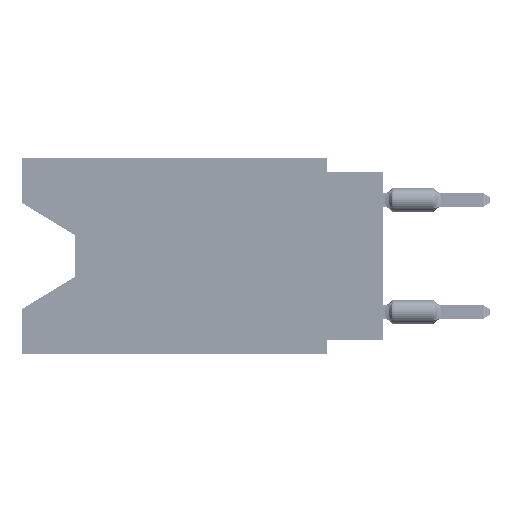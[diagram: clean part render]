
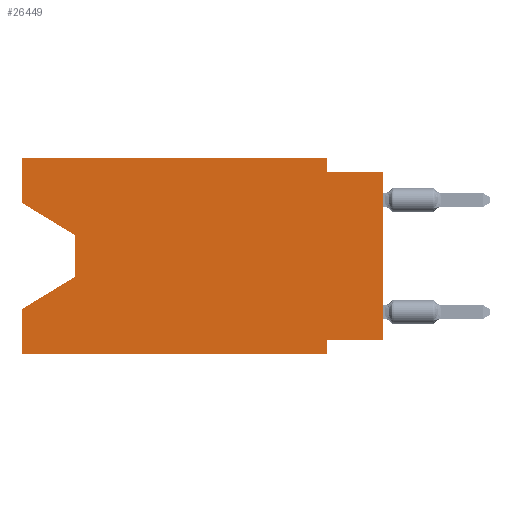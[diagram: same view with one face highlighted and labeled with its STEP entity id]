
A CAD part, left-side view. The second image highlights one B-rep face of the part: STEP entity #26449.
In plain terms, the highlighted planar face has unit normal (-1, 0, 0).
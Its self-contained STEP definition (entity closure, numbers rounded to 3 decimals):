
#415 = EDGE_CURVE ( 'NONE', #91928, #70264, #32800, .T. ) ;
#501 = VECTOR ( 'NONE', #87313, 1000. ) ;
#2110 = VERTEX_POINT ( 'NONE', #8948 ) ;
#2364 = AXIS2_PLACEMENT_3D ( 'NONE', #51618, #16560, #9546 ) ;
#3409 = EDGE_LOOP ( 'NONE', ( #31632, #90401, #66852, #14680, #78663, #9632, #33947, #86765, #17434, #77736, #16209, #39701 ) ) ;
#6005 = VECTOR ( 'NONE', #63480, 1000. ) ;
#6230 = LINE ( 'NONE', #7139, #47589 ) ;
#6502 = VERTEX_POINT ( 'NONE', #66421 ) ;
#6933 = VECTOR ( 'NONE', #83933, 1000. ) ;
#7139 = CARTESIAN_POINT ( 'NONE',  ( 0., 2.54, -8.89 ) ) ;
#7736 = LINE ( 'NONE', #29699, #42891 ) ;
#8948 = CARTESIAN_POINT ( 'NONE',  ( 0., 16.383, -6.852 ) ) ;
#8988 = CARTESIAN_POINT ( 'NONE',  ( 0., 16.383, -8.89 ) ) ;
#9546 = DIRECTION ( 'NONE',  ( 0., 0., -1. ) ) ;
#9632 = ORIENTED_EDGE ( 'NONE', *, *, #46198, .F. ) ;
#10314 = LINE ( 'NONE', #31351, #47722 ) ;
#10321 = EDGE_CURVE ( 'NONE', #17218, #91928, #56484, .T. ) ;
#10477 = VECTOR ( 'NONE', #26398, 1000. ) ;
#10602 = CARTESIAN_POINT ( 'NONE',  ( 0., 0., -8.255 ) ) ;
#10985 = LINE ( 'NONE', #24553, #40833 ) ;
#11067 = LINE ( 'NONE', #10602, #6933 ) ;
#11423 = EDGE_CURVE ( 'NONE', #24827, #88040, #52469, .T. ) ;
#13039 = EDGE_CURVE ( 'NONE', #65469, #24827, #7736, .T. ) ;
#13699 = DIRECTION ( 'NONE',  ( 0., 0., -1. ) ) ;
#14680 = ORIENTED_EDGE ( 'NONE', *, *, #41420, .F. ) ;
#16209 = ORIENTED_EDGE ( 'NONE', *, *, #34091, .F. ) ;
#16560 = DIRECTION ( 'NONE',  ( 1., 0., 0. ) ) ;
#17218 = VERTEX_POINT ( 'NONE', #73197 ) ;
#17265 = VECTOR ( 'NONE', #38890, 1000. ) ;
#17434 = ORIENTED_EDGE ( 'NONE', *, *, #11423, .F. ) ;
#23941 = LINE ( 'NONE', #8988, #33821 ) ;
#24316 = CARTESIAN_POINT ( 'NONE',  ( 0., 13.97, -5.385 ) ) ;
#24553 = CARTESIAN_POINT ( 'NONE',  ( 0., 16.383, 0. ) ) ;
#24827 = VERTEX_POINT ( 'NONE', #81122 ) ;
#26398 = DIRECTION ( 'NONE',  ( 0., 0.855, -0.519 ) ) ;
#26449 = ADVANCED_FACE ( 'NONE', ( #58167 ), #87581, .F. ) ;
#28841 = VERTEX_POINT ( 'NONE', #64454 ) ;
#28886 = CARTESIAN_POINT ( 'NONE',  ( 0., 16.383, -2.038 ) ) ;
#29564 = DIRECTION ( 'NONE',  ( 0., -1., 0. ) ) ;
#29699 = CARTESIAN_POINT ( 'NONE',  ( 0., 2.54, 0. ) ) ;
#30305 = LINE ( 'NONE', #31681, #501 ) ;
#31351 = CARTESIAN_POINT ( 'NONE',  ( 0., 0., 0. ) ) ;
#31632 = ORIENTED_EDGE ( 'NONE', *, *, #10321, .T. ) ;
#31681 = CARTESIAN_POINT ( 'NONE',  ( 0., 16.383, 0. ) ) ;
#32800 = LINE ( 'NONE', #61749, #65895 ) ;
#33802 = EDGE_CURVE ( 'NONE', #6502, #88040, #10314, .T. ) ;
#33821 = VECTOR ( 'NONE', #29564, 1000. ) ;
#33947 = ORIENTED_EDGE ( 'NONE', *, *, #63812, .F. ) ;
#34091 = EDGE_CURVE ( 'NONE', #28841, #65469, #42968, .T. ) ;
#34290 = CARTESIAN_POINT ( 'NONE',  ( 0., 2.54, 0. ) ) ;
#36263 = DIRECTION ( 'NONE',  ( 0., 0., -1. ) ) ;
#36564 = EDGE_CURVE ( 'NONE', #70264, #2110, #54462, .T. ) ;
#38890 = DIRECTION ( 'NONE',  ( 0., -1., 0. ) ) ;
#39701 = ORIENTED_EDGE ( 'NONE', *, *, #40265, .F. ) ;
#39791 = DIRECTION ( 'NONE',  ( 0., 0., -1. ) ) ;
#40265 = EDGE_CURVE ( 'NONE', #17218, #28841, #10985, .T. ) ;
#40833 = VECTOR ( 'NONE', #73633, 1000. ) ;
#41420 = EDGE_CURVE ( 'NONE', #46893, #2110, #30305, .T. ) ;
#42891 = VECTOR ( 'NONE', #36263, 1000. ) ;
#42968 = LINE ( 'NONE', #63541, #44571 ) ;
#44571 = VECTOR ( 'NONE', #78943, 1000. ) ;
#46198 = EDGE_CURVE ( 'NONE', #57644, #79376, #6230, .T. ) ;
#46893 = VERTEX_POINT ( 'NONE', #47148 ) ;
#47148 = CARTESIAN_POINT ( 'NONE',  ( 0., 16.383, -8.89 ) ) ;
#47589 = VECTOR ( 'NONE', #13699, 1000. ) ;
#47722 = VECTOR ( 'NONE', #65945, 1000. ) ;
#49917 = CARTESIAN_POINT ( 'NONE',  ( 0., 2.54, -8.89 ) ) ;
#51554 = CARTESIAN_POINT ( 'NONE',  ( 0., 2.54, -8.255 ) ) ;
#51618 = CARTESIAN_POINT ( 'NONE',  ( 0., 16.383, 0. ) ) ;
#52469 = LINE ( 'NONE', #80952, #17265 ) ;
#54462 = LINE ( 'NONE', #67530, #10477 ) ;
#56484 = LINE ( 'NONE', #28886, #6005 ) ;
#57644 = VERTEX_POINT ( 'NONE', #51554 ) ;
#58167 = FACE_OUTER_BOUND ( 'NONE', #3409, .T. ) ;
#61749 = CARTESIAN_POINT ( 'NONE',  ( 0., 13.97, -3.505 ) ) ;
#62169 = CARTESIAN_POINT ( 'NONE',  ( 0., 0., -0.635 ) ) ;
#63480 = DIRECTION ( 'NONE',  ( 0., -0.855, -0.519 ) ) ;
#63541 = CARTESIAN_POINT ( 'NONE',  ( 0., 16.383, 0. ) ) ;
#63812 = EDGE_CURVE ( 'NONE', #6502, #57644, #11067, .T. ) ;
#64454 = CARTESIAN_POINT ( 'NONE',  ( 0., 16.383, 0. ) ) ;
#65469 = VERTEX_POINT ( 'NONE', #34290 ) ;
#65574 = EDGE_CURVE ( 'NONE', #46893, #79376, #23941, .T. ) ;
#65895 = VECTOR ( 'NONE', #39791, 1000. ) ;
#65945 = DIRECTION ( 'NONE',  ( 0., 0., 1. ) ) ;
#66421 = CARTESIAN_POINT ( 'NONE',  ( 0., 0., -8.255 ) ) ;
#66852 = ORIENTED_EDGE ( 'NONE', *, *, #36564, .T. ) ;
#67530 = CARTESIAN_POINT ( 'NONE',  ( 0., 13.97, -5.385 ) ) ;
#70264 = VERTEX_POINT ( 'NONE', #24316 ) ;
#73197 = CARTESIAN_POINT ( 'NONE',  ( 0., 16.383, -2.038 ) ) ;
#73633 = DIRECTION ( 'NONE',  ( 0., 0., 1. ) ) ;
#76026 = CARTESIAN_POINT ( 'NONE',  ( 0., 13.97, -3.505 ) ) ;
#77736 = ORIENTED_EDGE ( 'NONE', *, *, #13039, .F. ) ;
#78663 = ORIENTED_EDGE ( 'NONE', *, *, #65574, .T. ) ;
#78943 = DIRECTION ( 'NONE',  ( 0., -1., 0. ) ) ;
#79376 = VERTEX_POINT ( 'NONE', #49917 ) ;
#80952 = CARTESIAN_POINT ( 'NONE',  ( 0., 0., -0.635 ) ) ;
#81122 = CARTESIAN_POINT ( 'NONE',  ( 0., 2.54, -0.635 ) ) ;
#83933 = DIRECTION ( 'NONE',  ( 0., 1., 0. ) ) ;
#86765 = ORIENTED_EDGE ( 'NONE', *, *, #33802, .T. ) ;
#87313 = DIRECTION ( 'NONE',  ( 0., 0., 1. ) ) ;
#87581 = PLANE ( 'NONE',  #2364 ) ;
#88040 = VERTEX_POINT ( 'NONE', #62169 ) ;
#90401 = ORIENTED_EDGE ( 'NONE', *, *, #415, .T. ) ;
#91928 = VERTEX_POINT ( 'NONE', #76026 ) ;
